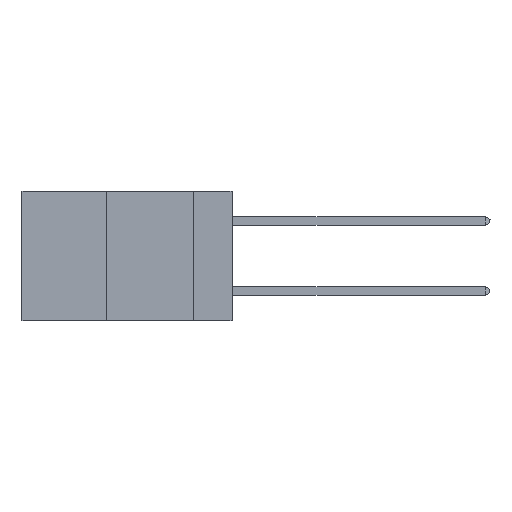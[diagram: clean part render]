
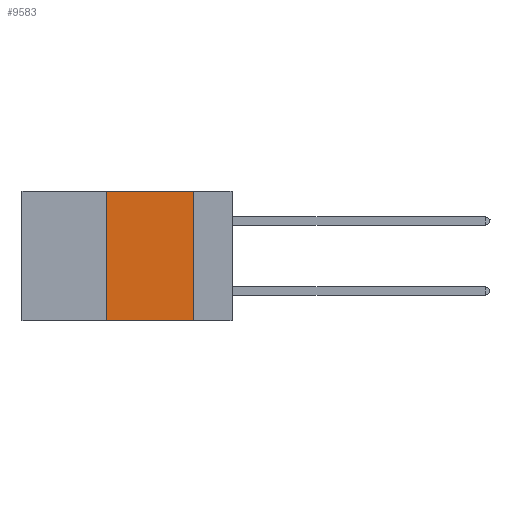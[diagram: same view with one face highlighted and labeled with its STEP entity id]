
A CAD part, left-side view. The second image highlights one B-rep face of the part: STEP entity #9583.
In plain terms, the highlighted planar face has unit normal (-1, 0, 0).
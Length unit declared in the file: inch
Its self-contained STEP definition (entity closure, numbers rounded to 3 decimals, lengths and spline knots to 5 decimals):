
#57 = VERTEX_POINT ( 'NONE', #5864 ) ;
#220 = CARTESIAN_POINT ( 'NONE',  ( 0., 0.11, 0. ) ) ;
#427 = DIRECTION ( 'NONE',  ( 1., 0., 0. ) ) ;
#725 = LINE ( 'NONE', #5726, #8781 ) ;
#789 = VERTEX_POINT ( 'NONE', #2466 ) ;
#1248 = PLANE ( 'NONE',  #6115 ) ;
#1296 = VERTEX_POINT ( 'NONE', #220 ) ;
#1316 = LINE ( 'NONE', #9535, #4401 ) ;
#1486 = EDGE_CURVE ( 'NONE', #4248, #789, #1316, .T. ) ;
#2025 = DIRECTION ( 'NONE',  ( 0., 0., -1. ) ) ;
#2106 = DIRECTION ( 'NONE',  ( 0., 0., -1. ) ) ;
#2466 = CARTESIAN_POINT ( 'NONE',  ( 0., 0.11, -0.37 ) ) ;
#3535 = ORIENTED_EDGE ( 'NONE', *, *, #4937, .F. ) ;
#4035 = DIRECTION ( 'NONE',  ( 0., 0., 1. ) ) ;
#4248 = VERTEX_POINT ( 'NONE', #5605 ) ;
#4401 = VECTOR ( 'NONE', #4732, 39.37008 ) ;
#4732 = DIRECTION ( 'NONE',  ( 0., -1., 0. ) ) ;
#4937 = EDGE_CURVE ( 'NONE', #57, #1296, #7750, .T. ) ;
#5200 = ORIENTED_EDGE ( 'NONE', *, *, #7052, .F. ) ;
#5341 = CARTESIAN_POINT ( 'NONE',  ( 0., 0.11, 0. ) ) ;
#5605 = CARTESIAN_POINT ( 'NONE',  ( 0., 0.36, -0.37 ) ) ;
#5726 = CARTESIAN_POINT ( 'NONE',  ( 0., 0.36, 0. ) ) ;
#5864 = CARTESIAN_POINT ( 'NONE',  ( 0., 0.36, 0. ) ) ;
#6115 = AXIS2_PLACEMENT_3D ( 'NONE', #7107, #427, #2106 ) ;
#6165 = LINE ( 'NONE', #5341, #10253 ) ;
#6289 = DIRECTION ( 'NONE',  ( 0., -1., 0. ) ) ;
#7052 = EDGE_CURVE ( 'NONE', #1296, #789, #6165, .T. ) ;
#7107 = CARTESIAN_POINT ( 'NONE',  ( 0., 0.6, 0. ) ) ;
#7654 = ORIENTED_EDGE ( 'NONE', *, *, #1486, .T. ) ;
#7750 = LINE ( 'NONE', #9519, #10304 ) ;
#7866 = ORIENTED_EDGE ( 'NONE', *, *, #10172, .F. ) ;
#8781 = VECTOR ( 'NONE', #4035, 39.37008 ) ;
#9519 = CARTESIAN_POINT ( 'NONE',  ( 0., 0.6, 0. ) ) ;
#9535 = CARTESIAN_POINT ( 'NONE',  ( 0., 0.6, -0.37 ) ) ;
#9583 = ADVANCED_FACE ( 'NONE', ( #10563 ), #1248, .F. ) ;
#10114 = EDGE_LOOP ( 'NONE', ( #5200, #3535, #7866, #7654 ) ) ;
#10172 = EDGE_CURVE ( 'NONE', #4248, #57, #725, .T. ) ;
#10253 = VECTOR ( 'NONE', #2025, 39.37008 ) ;
#10304 = VECTOR ( 'NONE', #6289, 39.37008 ) ;
#10563 = FACE_OUTER_BOUND ( 'NONE', #10114, .T. ) ;
